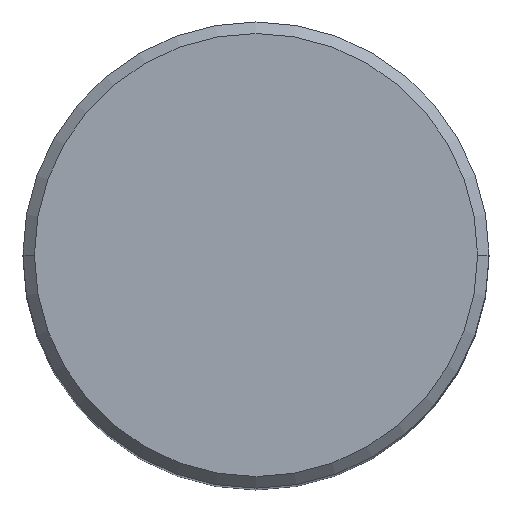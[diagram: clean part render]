
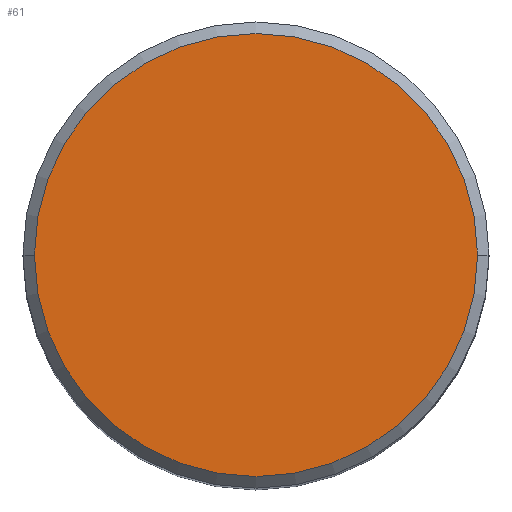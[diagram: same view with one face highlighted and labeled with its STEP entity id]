
A CAD part, top view. The second image highlights one B-rep face of the part: STEP entity #61.
In plain terms, the highlighted planar face has unit normal (0, 0, 1).
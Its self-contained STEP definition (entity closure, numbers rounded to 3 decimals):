
#1 = ORIENTED_EDGE ( 'NONE', *, *, #173, .T. ) ;
#23 = AXIS2_PLACEMENT_3D ( 'NONE', #154, #151, #141 ) ;
#34 = FACE_OUTER_BOUND ( 'NONE', #92, .T. ) ;
#60 = CIRCLE ( 'NONE', #71, 1.92 ) ;
#61 = ADVANCED_FACE ( 'NONE', ( #34 ), #192, .T. ) ;
#71 = AXIS2_PLACEMENT_3D ( 'NONE', #232, #222, #87 ) ;
#75 = VERTEX_POINT ( 'NONE', #207 ) ;
#85 = AXIS2_PLACEMENT_3D ( 'NONE', #160, #203, #205 ) ;
#87 = DIRECTION ( 'NONE',  ( 1., 0., 0. ) ) ;
#92 = EDGE_LOOP ( 'NONE', ( #1, #211 ) ) ;
#112 = CARTESIAN_POINT ( 'NONE',  ( -1.92, 0., 9.32 ) ) ;
#139 = EDGE_CURVE ( 'NONE', #75, #220, #60, .T. ) ;
#141 = DIRECTION ( 'NONE',  ( 1., 0., 0. ) ) ;
#151 = DIRECTION ( 'NONE',  ( 0., 0., 1. ) ) ;
#154 = CARTESIAN_POINT ( 'NONE',  ( 0., 0., 9.32 ) ) ;
#160 = CARTESIAN_POINT ( 'NONE',  ( 0., 0., 9.32 ) ) ;
#173 = EDGE_CURVE ( 'NONE', #220, #75, #226, .T. ) ;
#192 = PLANE ( 'NONE',  #85 ) ;
#203 = DIRECTION ( 'NONE',  ( 0., 0., 1. ) ) ;
#205 = DIRECTION ( 'NONE',  ( 1., 0., 0. ) ) ;
#207 = CARTESIAN_POINT ( 'NONE',  ( 1.92, 0., 9.32 ) ) ;
#211 = ORIENTED_EDGE ( 'NONE', *, *, #139, .T. ) ;
#220 = VERTEX_POINT ( 'NONE', #112 ) ;
#222 = DIRECTION ( 'NONE',  ( 0., 0., 1. ) ) ;
#226 = CIRCLE ( 'NONE', #23, 1.92 ) ;
#232 = CARTESIAN_POINT ( 'NONE',  ( 0., 0., 9.32 ) ) ;
